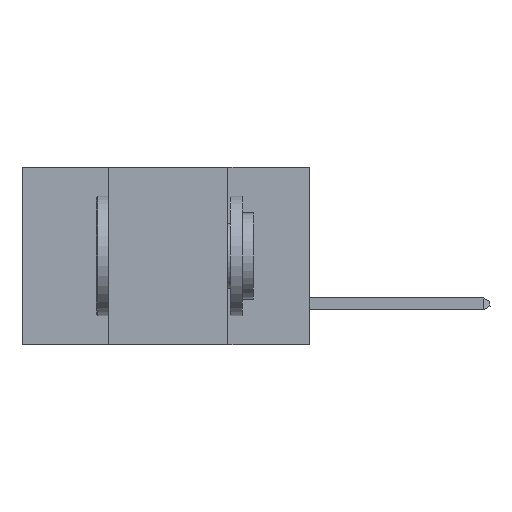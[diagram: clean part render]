
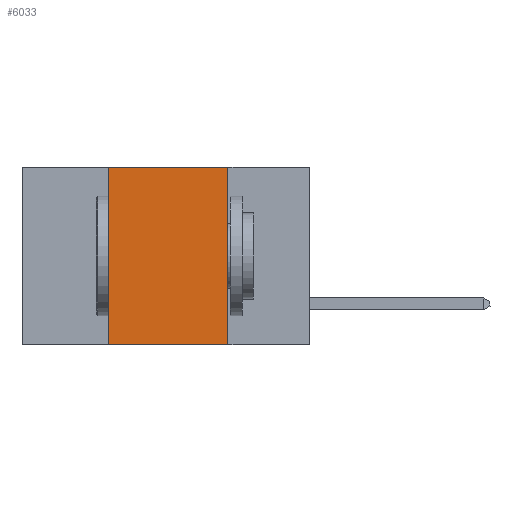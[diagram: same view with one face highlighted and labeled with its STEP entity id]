
A CAD part, left-side view. The second image highlights one B-rep face of the part: STEP entity #6033.
In plain terms, the highlighted planar face has unit normal (-1, 0, 0).
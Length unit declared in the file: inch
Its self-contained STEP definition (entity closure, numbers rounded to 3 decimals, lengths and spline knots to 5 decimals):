
#192 = DIRECTION ( 'NONE',  ( 0., 0., -1. ) ) ;
#753 = LINE ( 'NONE', #6185, #7476 ) ;
#992 = CARTESIAN_POINT ( 'NONE',  ( 0., 0.17, -0.37 ) ) ;
#1618 = VERTEX_POINT ( 'NONE', #4923 ) ;
#1660 = VECTOR ( 'NONE', #2460, 39.37008 ) ;
#1772 = VERTEX_POINT ( 'NONE', #2868 ) ;
#1815 = ORIENTED_EDGE ( 'NONE', *, *, #9552, .F. ) ;
#2062 = EDGE_CURVE ( 'NONE', #1618, #3469, #8605, .T. ) ;
#2460 = DIRECTION ( 'NONE',  ( 0., 0., 1. ) ) ;
#2868 = CARTESIAN_POINT ( 'NONE',  ( 0., 0.17, 0. ) ) ;
#3042 = DIRECTION ( 'NONE',  ( 1., 0., 0. ) ) ;
#3224 = DIRECTION ( 'NONE',  ( 0., -1., 0. ) ) ;
#3340 = VECTOR ( 'NONE', #9254, 39.37008 ) ;
#3469 = VERTEX_POINT ( 'NONE', #8853 ) ;
#4923 = CARTESIAN_POINT ( 'NONE',  ( 0., 0.42, -0.37 ) ) ;
#5292 = EDGE_LOOP ( 'NONE', ( #8323, #1815, #7976, #6478 ) ) ;
#5368 = PLANE ( 'NONE',  #6217 ) ;
#5924 = FACE_OUTER_BOUND ( 'NONE', #5292, .T. ) ;
#6033 = ADVANCED_FACE ( 'NONE', ( #5924 ), #5368, .F. ) ;
#6130 = VECTOR ( 'NONE', #3224, 39.37008 ) ;
#6185 = CARTESIAN_POINT ( 'NONE',  ( 0., 0.6, 0. ) ) ;
#6217 = AXIS2_PLACEMENT_3D ( 'NONE', #8246, #3042, #192 ) ;
#6307 = DIRECTION ( 'NONE',  ( 0., -1., 0. ) ) ;
#6478 = ORIENTED_EDGE ( 'NONE', *, *, #9067, .T. ) ;
#6879 = CARTESIAN_POINT ( 'NONE',  ( 0., 0.6, -0.37 ) ) ;
#6882 = CARTESIAN_POINT ( 'NONE',  ( 0., 0.42, 0. ) ) ;
#7231 = EDGE_CURVE ( 'NONE', #1772, #9006, #7747, .T. ) ;
#7476 = VECTOR ( 'NONE', #6307, 39.37008 ) ;
#7691 = CARTESIAN_POINT ( 'NONE',  ( 0., 0.17, 0. ) ) ;
#7747 = LINE ( 'NONE', #7691, #3340 ) ;
#7976 = ORIENTED_EDGE ( 'NONE', *, *, #2062, .F. ) ;
#8246 = CARTESIAN_POINT ( 'NONE',  ( 0., 0.6, 0. ) ) ;
#8323 = ORIENTED_EDGE ( 'NONE', *, *, #7231, .F. ) ;
#8605 = LINE ( 'NONE', #6882, #1660 ) ;
#8853 = CARTESIAN_POINT ( 'NONE',  ( 0., 0.42, 0. ) ) ;
#9006 = VERTEX_POINT ( 'NONE', #992 ) ;
#9067 = EDGE_CURVE ( 'NONE', #1618, #9006, #9119, .T. ) ;
#9119 = LINE ( 'NONE', #6879, #6130 ) ;
#9254 = DIRECTION ( 'NONE',  ( 0., 0., -1. ) ) ;
#9552 = EDGE_CURVE ( 'NONE', #3469, #1772, #753, .T. ) ;
